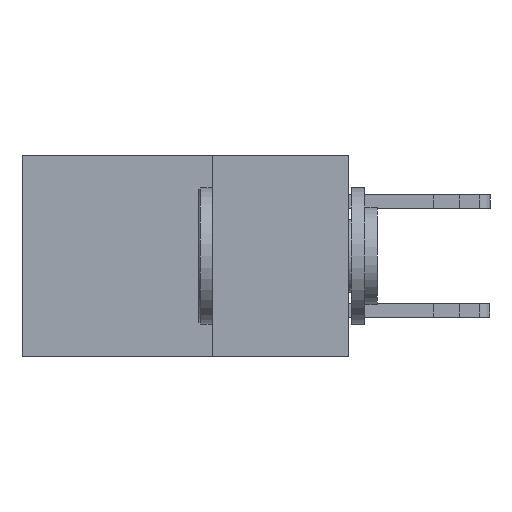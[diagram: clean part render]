
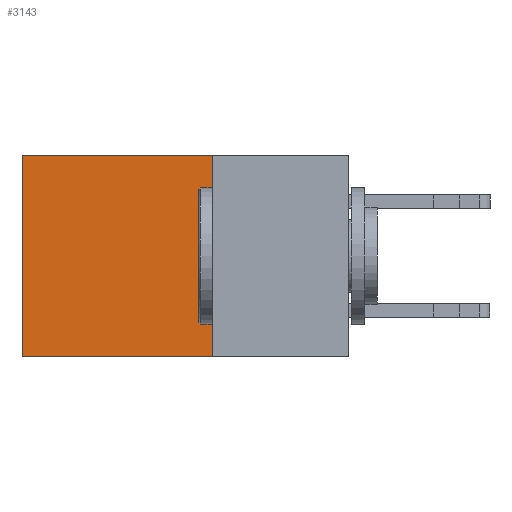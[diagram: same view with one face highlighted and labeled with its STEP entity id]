
A CAD part, left-side view. The second image highlights one B-rep face of the part: STEP entity #3143.
In plain terms, the highlighted planar face has unit normal (-1, 0, 0).
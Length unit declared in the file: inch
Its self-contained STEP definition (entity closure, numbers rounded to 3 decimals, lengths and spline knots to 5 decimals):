
#800 = EDGE_LOOP ( 'NONE', ( #7688, #17548, #10293, #9073 ) ) ;
#3136 = LINE ( 'NONE', #13657, #17350 ) ;
#3143 = ADVANCED_FACE ( 'NONE', ( #15671 ), #16994, .F. ) ;
#3411 = VERTEX_POINT ( 'NONE', #12973 ) ;
#3707 = VERTEX_POINT ( 'NONE', #7031 ) ;
#4463 = LINE ( 'NONE', #17544, #11523 ) ;
#4496 = CARTESIAN_POINT ( 'NONE',  ( 0.298, 0.6, 0. ) ) ;
#4619 = EDGE_CURVE ( 'NONE', #3411, #5698, #7529, .T. ) ;
#5698 = VERTEX_POINT ( 'NONE', #15713 ) ;
#7031 = CARTESIAN_POINT ( 'NONE',  ( 0.298, 0.25, 0. ) ) ;
#7201 = DIRECTION ( 'NONE',  ( 0., 0., -1. ) ) ;
#7529 = LINE ( 'NONE', #9755, #11275 ) ;
#7688 = ORIENTED_EDGE ( 'NONE', *, *, #13680, .T. ) ;
#9073 = ORIENTED_EDGE ( 'NONE', *, *, #11031, .T. ) ;
#9442 = EDGE_CURVE ( 'NONE', #3707, #3411, #3136, .T. ) ;
#9755 = CARTESIAN_POINT ( 'NONE',  ( 0.298, 0.25, -0.37 ) ) ;
#10293 = ORIENTED_EDGE ( 'NONE', *, *, #9442, .F. ) ;
#10467 = DIRECTION ( 'NONE',  ( 0., 1., 0. ) ) ;
#11031 = EDGE_CURVE ( 'NONE', #3707, #16732, #4463, .T. ) ;
#11275 = VECTOR ( 'NONE', #11543, 39.37008 ) ;
#11523 = VECTOR ( 'NONE', #10467, 39.37008 ) ;
#11543 = DIRECTION ( 'NONE',  ( 0., 1., 0. ) ) ;
#12060 = VECTOR ( 'NONE', #7201, 39.37008 ) ;
#12973 = CARTESIAN_POINT ( 'NONE',  ( 0.298, 0.25, -0.37 ) ) ;
#13657 = CARTESIAN_POINT ( 'NONE',  ( 0.298, 0.25, 0. ) ) ;
#13680 = EDGE_CURVE ( 'NONE', #16732, #5698, #15916, .T. ) ;
#14250 = AXIS2_PLACEMENT_3D ( 'NONE', #14625, #14585, #14565 ) ;
#14294 = CARTESIAN_POINT ( 'NONE',  ( 0.298, 0.6, 0. ) ) ;
#14565 = DIRECTION ( 'NONE',  ( 0., 0., -1. ) ) ;
#14585 = DIRECTION ( 'NONE',  ( 1., 0., 0. ) ) ;
#14625 = CARTESIAN_POINT ( 'NONE',  ( 0.298, 0.25, 0. ) ) ;
#15671 = FACE_OUTER_BOUND ( 'NONE', #800, .T. ) ;
#15713 = CARTESIAN_POINT ( 'NONE',  ( 0.298, 0.6, -0.37 ) ) ;
#15916 = LINE ( 'NONE', #14294, #12060 ) ;
#16498 = DIRECTION ( 'NONE',  ( 0., 0., -1. ) ) ;
#16732 = VERTEX_POINT ( 'NONE', #4496 ) ;
#16994 = PLANE ( 'NONE',  #14250 ) ;
#17350 = VECTOR ( 'NONE', #16498, 39.37008 ) ;
#17544 = CARTESIAN_POINT ( 'NONE',  ( 0.298, 0.25, 0. ) ) ;
#17548 = ORIENTED_EDGE ( 'NONE', *, *, #4619, .F. ) ;
